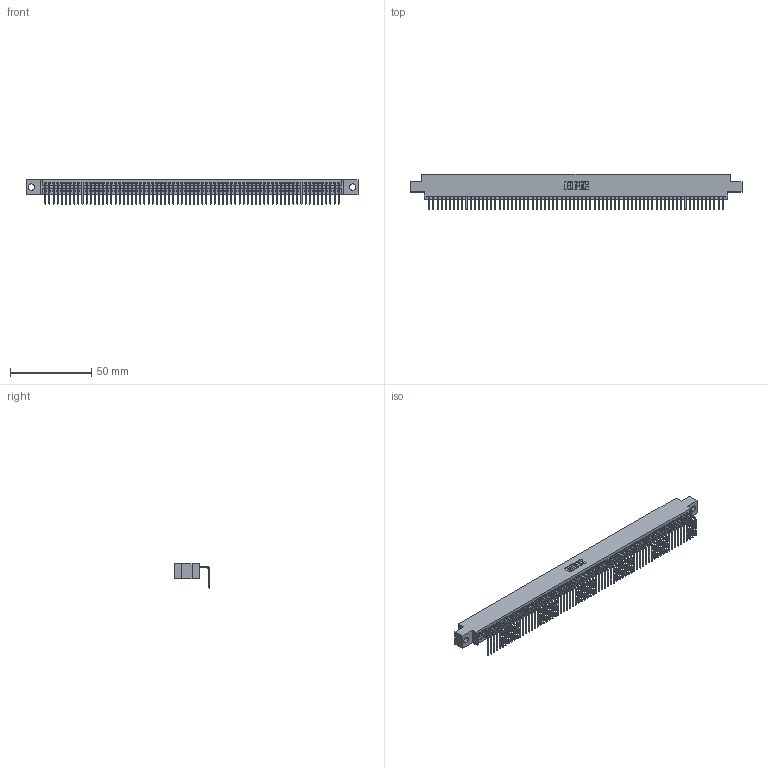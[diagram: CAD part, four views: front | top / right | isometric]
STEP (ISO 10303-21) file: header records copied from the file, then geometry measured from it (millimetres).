
FILE_DESCRIPTION (( 'STEP AP203' ), '1' );
FILE_NAME ('395-072-558-604.STEP', '2021-06-11T20:22:52', ( '' ), ( '' ), 'SwSTEP 2.0', 'SolidWorks 2020', '' );
FILE_SCHEMA (( 'CONFIG_CONTROL_DESIGN' ));
Length unit declared in the file: inch
Products named in the file (3): 345-292-001_558 Tail - 2; 395-072-558-604; 345 Part_0.170 Offset - 0.156 Dia-TI
Assembly tree (73 placements, depth 2):
  395-072-558-604
    345 Part_0.170 Offset - 0.156 Dia-TI
    345-292-001_558 Tail - 2  x72
Bounding box: 204.09 x 21.83 x 15.37 mm (x, y, z)
Volume: 19650.9 mm3; surface area: 27900.6 mm2
Topology: 73 solids, 73 shells, 4464 faces, 13493 edges, 8898 vertices
Faces by surface type: plane 3122, cylinder 1342
Entity records: 50785 total; most frequent: ORIENTED_EDGE 8810, CARTESIAN_POINT 8806, DIRECTION 7645, EDGE_CURVE 4405, VECTOR 3985, LINE 3985, VERTEX_POINT 2934, AXIS2_PLACEMENT_3D 1830
